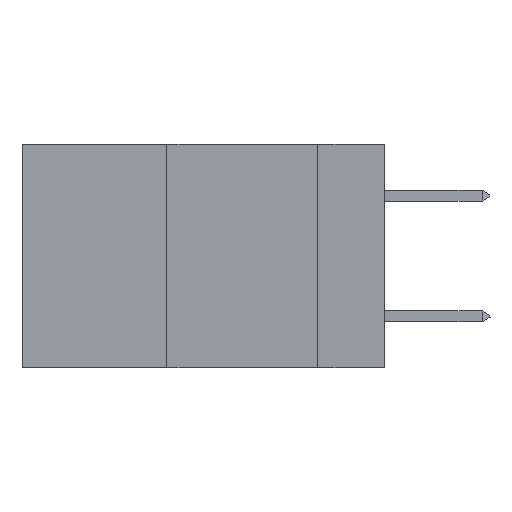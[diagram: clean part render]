
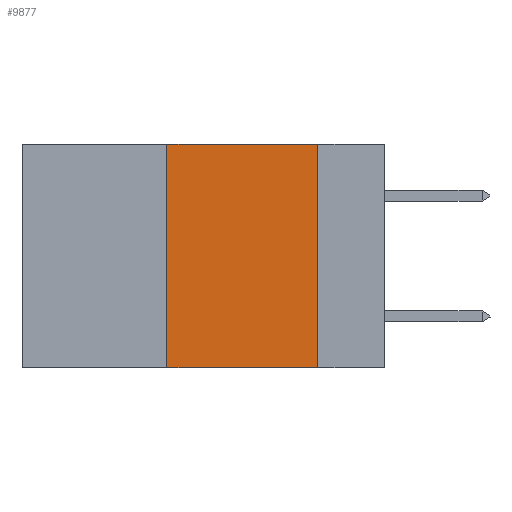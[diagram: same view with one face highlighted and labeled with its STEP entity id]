
A CAD part, left-side view. The second image highlights one B-rep face of the part: STEP entity #9877.
In plain terms, the highlighted planar face has unit normal (-1, 0, 0).
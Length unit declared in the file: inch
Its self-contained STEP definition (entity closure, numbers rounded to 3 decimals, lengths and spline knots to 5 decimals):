
#404 = EDGE_CURVE ( 'NONE', #12430, #25093, #3915, .T. ) ;
#1149 = EDGE_LOOP ( 'NONE', ( #17987, #8270, #9190, #14265 ) ) ;
#3915 = LINE ( 'NONE', #14010, #16389 ) ;
#4558 = VECTOR ( 'NONE', #6880, 39.37008 ) ;
#4562 = EDGE_CURVE ( 'NONE', #23280, #20938, #24085, .T. ) ;
#5689 = VECTOR ( 'NONE', #19399, 39.37008 ) ;
#6618 = CARTESIAN_POINT ( 'NONE',  ( 0., 0.36, 0. ) ) ;
#6880 = DIRECTION ( 'NONE',  ( 0., 0., 1. ) ) ;
#7179 = DIRECTION ( 'NONE',  ( 0., 0., -1. ) ) ;
#8270 = ORIENTED_EDGE ( 'NONE', *, *, #20434, .F. ) ;
#8818 = CARTESIAN_POINT ( 'NONE',  ( 0., 0.11, 0. ) ) ;
#9096 = LINE ( 'NONE', #9470, #15486 ) ;
#9190 = ORIENTED_EDGE ( 'NONE', *, *, #4562, .F. ) ;
#9470 = CARTESIAN_POINT ( 'NONE',  ( 0., 0.6, 0. ) ) ;
#9877 = ADVANCED_FACE ( 'NONE', ( #24755 ), #11012, .F. ) ;
#11012 = PLANE ( 'NONE',  #21784 ) ;
#11601 = CARTESIAN_POINT ( 'NONE',  ( 0., 0.36, -0.37 ) ) ;
#12430 = VERTEX_POINT ( 'NONE', #8818 ) ;
#13173 = DIRECTION ( 'NONE',  ( 1., 0., 0. ) ) ;
#13920 = LINE ( 'NONE', #23354, #5689 ) ;
#14010 = CARTESIAN_POINT ( 'NONE',  ( 0., 0.11, 0. ) ) ;
#14265 = ORIENTED_EDGE ( 'NONE', *, *, #20514, .T. ) ;
#15087 = CARTESIAN_POINT ( 'NONE',  ( 0., 0.6, 0. ) ) ;
#15486 = VECTOR ( 'NONE', #22847, 39.37008 ) ;
#16389 = VECTOR ( 'NONE', #23558, 39.37008 ) ;
#17987 = ORIENTED_EDGE ( 'NONE', *, *, #404, .F. ) ;
#19399 = DIRECTION ( 'NONE',  ( 0., -1., 0. ) ) ;
#20434 = EDGE_CURVE ( 'NONE', #20938, #12430, #9096, .T. ) ;
#20514 = EDGE_CURVE ( 'NONE', #23280, #25093, #13920, .T. ) ;
#20938 = VERTEX_POINT ( 'NONE', #23452 ) ;
#21784 = AXIS2_PLACEMENT_3D ( 'NONE', #15087, #13173, #7179 ) ;
#22847 = DIRECTION ( 'NONE',  ( 0., -1., 0. ) ) ;
#23280 = VERTEX_POINT ( 'NONE', #11601 ) ;
#23316 = CARTESIAN_POINT ( 'NONE',  ( 0., 0.11, -0.37 ) ) ;
#23354 = CARTESIAN_POINT ( 'NONE',  ( 0., 0.6, -0.37 ) ) ;
#23452 = CARTESIAN_POINT ( 'NONE',  ( 0., 0.36, 0. ) ) ;
#23558 = DIRECTION ( 'NONE',  ( 0., 0., -1. ) ) ;
#24085 = LINE ( 'NONE', #6618, #4558 ) ;
#24755 = FACE_OUTER_BOUND ( 'NONE', #1149, .T. ) ;
#25093 = VERTEX_POINT ( 'NONE', #23316 ) ;
